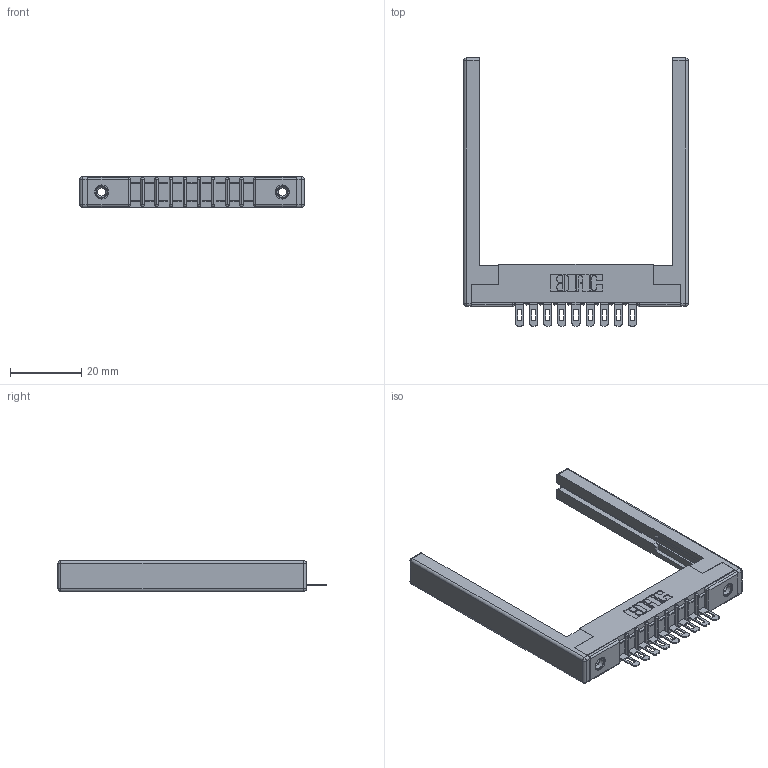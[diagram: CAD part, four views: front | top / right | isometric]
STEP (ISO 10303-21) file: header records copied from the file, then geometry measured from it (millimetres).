
FILE_DESCRIPTION (( 'STEP AP203' ), '1' );
FILE_NAME ('357-009-501-168.STEP', '2019-09-16T17:58:27', ( '' ), ( '' ), 'SwSTEP 2.0', 'SolidWorks 2016', '' );
FILE_SCHEMA (( 'CONFIG_CONTROL_DESIGN' ));
Length unit declared in the file: inch
Products named in the file (5): 307 Part_.156 Dia Mounting Holes; 307-290-002_501; 357-009-501-168; 307-220-068; 345-250-001_345-250-001-102
Assembly tree (14 placements, depth 2):
  357-009-501-168
    307 Part_.156 Dia Mounting Holes
    307-290-002_501  x9
    307-220-068  x2
    345-250-001_345-250-001-102  x2
Bounding box: 63.09 x 75.39 x 8.71 mm (x, y, z)
Volume: 8725.1 mm3; surface area: 10936.2 mm2
Topology: 14 solids, 14 shells, 966 faces, 2855 edges, 1854 vertices
Faces by surface type: plane 554, cylinder 368, sphere 28, cone 12, torus 4
Entity records: 15337 total; most frequent: CARTESIAN_POINT 2545, ORIENTED_EDGE 2524, DIRECTION 2510, EDGE_CURVE 1262, VECTOR 944, LINE 944, VERTEX_POINT 818, AXIS2_PLACEMENT_3D 783
